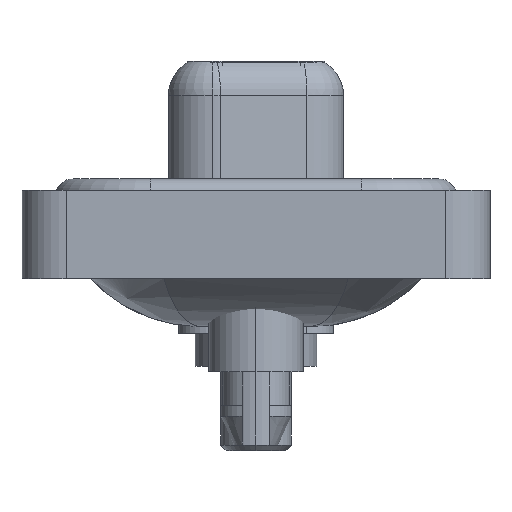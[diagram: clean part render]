
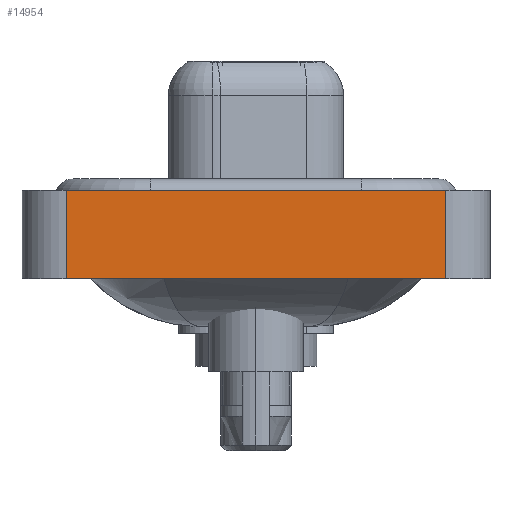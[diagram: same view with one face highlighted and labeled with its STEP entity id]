
A CAD part, left-side view. The second image highlights one B-rep face of the part: STEP entity #14954.
In plain terms, the highlighted planar face has unit normal (-1, 0, 0).
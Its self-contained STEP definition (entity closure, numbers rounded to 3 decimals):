
#427 = CARTESIAN_POINT ( 'NONE',  ( -7.3, -8.55, -3.6 ) ) ;
#618 = LINE ( 'NONE', #10836, #16738 ) ;
#674 = VERTEX_POINT ( 'NONE', #4295 ) ;
#702 = ORIENTED_EDGE ( 'NONE', *, *, #14738, .T. ) ;
#829 = DIRECTION ( 'NONE',  ( 0., 0., 1. ) ) ;
#2071 = DIRECTION ( 'NONE',  ( 0., 0., 1. ) ) ;
#2427 = VERTEX_POINT ( 'NONE', #11113 ) ;
#2677 = CARTESIAN_POINT ( 'NONE',  ( -7.3, -8.55, 0.4 ) ) ;
#3210 = VERTEX_POINT ( 'NONE', #427 ) ;
#3433 = LINE ( 'NONE', #13624, #3926 ) ;
#3926 = VECTOR ( 'NONE', #2071, 1000. ) ;
#4259 = VECTOR ( 'NONE', #17467, 1000. ) ;
#4295 = CARTESIAN_POINT ( 'NONE',  ( -7.3, 8.55, -3.6 ) ) ;
#4312 = CARTESIAN_POINT ( 'NONE',  ( -7.3, -8.55, -3.6 ) ) ;
#5148 = VERTEX_POINT ( 'NONE', #2677 ) ;
#5742 = DIRECTION ( 'NONE',  ( 0., -1., 0. ) ) ;
#5750 = EDGE_LOOP ( 'NONE', ( #11481, #11260, #10003, #702 ) ) ;
#7400 = EDGE_CURVE ( 'NONE', #3210, #5148, #3433, .T. ) ;
#8559 = VECTOR ( 'NONE', #5742, 1000. ) ;
#9454 = CARTESIAN_POINT ( 'NONE',  ( -7.3, -8.55, -3.6 ) ) ;
#9825 = PLANE ( 'NONE',  #10962 ) ;
#10003 = ORIENTED_EDGE ( 'NONE', *, *, #17431, .F. ) ;
#10304 = LINE ( 'NONE', #4312, #4259 ) ;
#10556 = DIRECTION ( 'NONE',  ( 0., 0., 1. ) ) ;
#10836 = CARTESIAN_POINT ( 'NONE',  ( -7.3, 8.55, -3.6 ) ) ;
#10962 = AXIS2_PLACEMENT_3D ( 'NONE', #9454, #14007, #829 ) ;
#11113 = CARTESIAN_POINT ( 'NONE',  ( -7.3, 8.55, 0.4 ) ) ;
#11260 = ORIENTED_EDGE ( 'NONE', *, *, #15918, .F. ) ;
#11481 = ORIENTED_EDGE ( 'NONE', *, *, #7400, .T. ) ;
#11827 = CARTESIAN_POINT ( 'NONE',  ( -7.3, -8.55, 0.4 ) ) ;
#13624 = CARTESIAN_POINT ( 'NONE',  ( -7.3, -8.55, -3.6 ) ) ;
#14007 = DIRECTION ( 'NONE',  ( -1., 0., 0. ) ) ;
#14738 = EDGE_CURVE ( 'NONE', #674, #3210, #10304, .T. ) ;
#14954 = ADVANCED_FACE ( 'NONE', ( #16698 ), #9825, .T. ) ;
#15918 = EDGE_CURVE ( 'NONE', #2427, #5148, #18529, .T. ) ;
#16698 = FACE_OUTER_BOUND ( 'NONE', #5750, .T. ) ;
#16738 = VECTOR ( 'NONE', #10556, 1000. ) ;
#17431 = EDGE_CURVE ( 'NONE', #674, #2427, #618, .T. ) ;
#17467 = DIRECTION ( 'NONE',  ( 0., -1., 0. ) ) ;
#18529 = LINE ( 'NONE', #11827, #8559 ) ;
